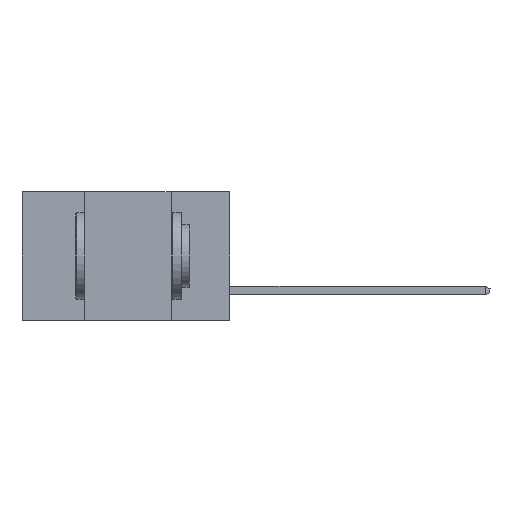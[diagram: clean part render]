
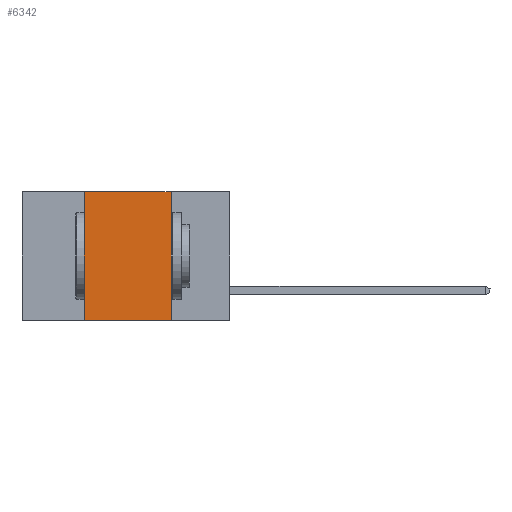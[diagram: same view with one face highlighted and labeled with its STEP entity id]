
A CAD part, left-side view. The second image highlights one B-rep face of the part: STEP entity #6342.
In plain terms, the highlighted planar face has unit normal (-1, 0, 0).
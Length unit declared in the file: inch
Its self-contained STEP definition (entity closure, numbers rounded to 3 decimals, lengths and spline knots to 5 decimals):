
#275 = ORIENTED_EDGE ( 'NONE', *, *, #3931, .T. ) ;
#605 = CARTESIAN_POINT ( 'NONE',  ( 0., 0.6, -0.37 ) ) ;
#644 = CARTESIAN_POINT ( 'NONE',  ( 0., 0.17, -0.37 ) ) ;
#892 = VERTEX_POINT ( 'NONE', #4956 ) ;
#1074 = LINE ( 'NONE', #605, #7044 ) ;
#1434 = EDGE_CURVE ( 'NONE', #10656, #1943, #6337, .T. ) ;
#1712 = DIRECTION ( 'NONE',  ( 0., 0., -1. ) ) ;
#1943 = VERTEX_POINT ( 'NONE', #644 ) ;
#3197 = ORIENTED_EDGE ( 'NONE', *, *, #6030, .F. ) ;
#3931 = EDGE_CURVE ( 'NONE', #12722, #1943, #1074, .T. ) ;
#4285 = EDGE_LOOP ( 'NONE', ( #9686, #3197, #8622, #275 ) ) ;
#4393 = CARTESIAN_POINT ( 'NONE',  ( 0., 0.17, 0. ) ) ;
#4875 = CARTESIAN_POINT ( 'NONE',  ( 0., 0.42, 0. ) ) ;
#4956 = CARTESIAN_POINT ( 'NONE',  ( 0., 0.42, 0. ) ) ;
#5575 = EDGE_CURVE ( 'NONE', #12722, #892, #12791, .T. ) ;
#6030 = EDGE_CURVE ( 'NONE', #892, #10656, #11783, .T. ) ;
#6131 = DIRECTION ( 'NONE',  ( 0., 0., -1. ) ) ;
#6337 = LINE ( 'NONE', #14882, #11734 ) ;
#6342 = ADVANCED_FACE ( 'NONE', ( #7639 ), #10316, .F. ) ;
#6367 = DIRECTION ( 'NONE',  ( 1., 0., 0. ) ) ;
#7044 = VECTOR ( 'NONE', #14645, 39.37008 ) ;
#7639 = FACE_OUTER_BOUND ( 'NONE', #4285, .T. ) ;
#8622 = ORIENTED_EDGE ( 'NONE', *, *, #5575, .F. ) ;
#9686 = ORIENTED_EDGE ( 'NONE', *, *, #1434, .F. ) ;
#10316 = PLANE ( 'NONE',  #10946 ) ;
#10656 = VERTEX_POINT ( 'NONE', #4393 ) ;
#10946 = AXIS2_PLACEMENT_3D ( 'NONE', #14222, #6367, #1712 ) ;
#10995 = VECTOR ( 'NONE', #12657, 39.37008 ) ;
#11734 = VECTOR ( 'NONE', #6131, 39.37008 ) ;
#11783 = LINE ( 'NONE', #12191, #12981 ) ;
#12191 = CARTESIAN_POINT ( 'NONE',  ( 0., 0.6, 0. ) ) ;
#12230 = CARTESIAN_POINT ( 'NONE',  ( 0., 0.42, -0.37 ) ) ;
#12657 = DIRECTION ( 'NONE',  ( 0., 0., 1. ) ) ;
#12722 = VERTEX_POINT ( 'NONE', #12230 ) ;
#12791 = LINE ( 'NONE', #4875, #10995 ) ;
#12981 = VECTOR ( 'NONE', #14641, 39.37008 ) ;
#14222 = CARTESIAN_POINT ( 'NONE',  ( 0., 0.6, 0. ) ) ;
#14641 = DIRECTION ( 'NONE',  ( 0., -1., 0. ) ) ;
#14645 = DIRECTION ( 'NONE',  ( 0., -1., 0. ) ) ;
#14882 = CARTESIAN_POINT ( 'NONE',  ( 0., 0.17, 0. ) ) ;
